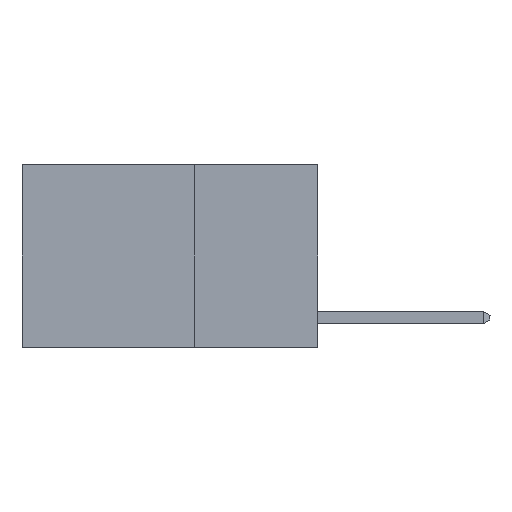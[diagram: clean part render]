
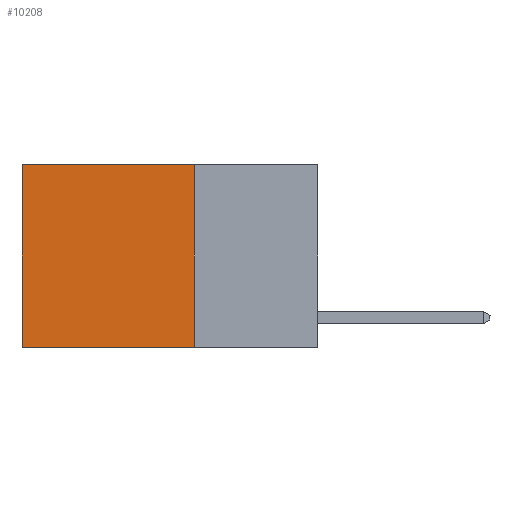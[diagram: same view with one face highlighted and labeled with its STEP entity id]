
A CAD part, left-side view. The second image highlights one B-rep face of the part: STEP entity #10208.
In plain terms, the highlighted planar face has unit normal (-1, 0, 0).
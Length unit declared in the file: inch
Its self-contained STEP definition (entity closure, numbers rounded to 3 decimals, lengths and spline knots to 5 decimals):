
#796 = LINE ( 'NONE', #3553, #7300 ) ;
#932 = VERTEX_POINT ( 'NONE', #9899 ) ;
#1137 = VECTOR ( 'NONE', #1715, 39.37008 ) ;
#1158 = LINE ( 'NONE', #10447, #4116 ) ;
#1715 = DIRECTION ( 'NONE',  ( 0., 0., -1. ) ) ;
#1800 = CARTESIAN_POINT ( 'NONE',  ( 0.2625, 0.25, 0. ) ) ;
#2267 = LINE ( 'NONE', #8555, #8526 ) ;
#2397 = DIRECTION ( 'NONE',  ( 1., 0., 0. ) ) ;
#3430 = EDGE_CURVE ( 'NONE', #6355, #932, #2267, .T. ) ;
#3553 = CARTESIAN_POINT ( 'NONE',  ( 0.2625, 0.6, 0. ) ) ;
#3679 = ORIENTED_EDGE ( 'NONE', *, *, #3430, .T. ) ;
#3944 = PLANE ( 'NONE',  #4107 ) ;
#4002 = FACE_OUTER_BOUND ( 'NONE', #10683, .T. ) ;
#4107 = AXIS2_PLACEMENT_3D ( 'NONE', #7612, #2397, #5086 ) ;
#4116 = VECTOR ( 'NONE', #8551, 39.37008 ) ;
#5086 = DIRECTION ( 'NONE',  ( 0., 0., -1. ) ) ;
#5306 = EDGE_CURVE ( 'NONE', #6355, #10913, #8979, .T. ) ;
#5366 = EDGE_CURVE ( 'NONE', #932, #8522, #796, .T. ) ;
#6355 = VERTEX_POINT ( 'NONE', #1800 ) ;
#6560 = CARTESIAN_POINT ( 'NONE',  ( 0.2625, 0.25, -0.37 ) ) ;
#6925 = ORIENTED_EDGE ( 'NONE', *, *, #5366, .T. ) ;
#7300 = VECTOR ( 'NONE', #10950, 39.37008 ) ;
#7612 = CARTESIAN_POINT ( 'NONE',  ( 0.2625, 0.25, 0. ) ) ;
#7735 = DIRECTION ( 'NONE',  ( 0., 1., 0. ) ) ;
#8126 = CARTESIAN_POINT ( 'NONE',  ( 0.2625, 0.6, -0.37 ) ) ;
#8301 = ORIENTED_EDGE ( 'NONE', *, *, #10554, .F. ) ;
#8522 = VERTEX_POINT ( 'NONE', #8126 ) ;
#8526 = VECTOR ( 'NONE', #7735, 39.37008 ) ;
#8551 = DIRECTION ( 'NONE',  ( 0., 1., 0. ) ) ;
#8555 = CARTESIAN_POINT ( 'NONE',  ( 0.2625, 0.25, 0. ) ) ;
#8979 = LINE ( 'NONE', #10892, #1137 ) ;
#9899 = CARTESIAN_POINT ( 'NONE',  ( 0.2625, 0.6, 0. ) ) ;
#10208 = ADVANCED_FACE ( 'NONE', ( #4002 ), #3944, .F. ) ;
#10447 = CARTESIAN_POINT ( 'NONE',  ( 0.2625, 0.25, -0.37 ) ) ;
#10554 = EDGE_CURVE ( 'NONE', #10913, #8522, #1158, .T. ) ;
#10683 = EDGE_LOOP ( 'NONE', ( #6925, #8301, #11391, #3679 ) ) ;
#10892 = CARTESIAN_POINT ( 'NONE',  ( 0.2625, 0.25, 0. ) ) ;
#10913 = VERTEX_POINT ( 'NONE', #6560 ) ;
#10950 = DIRECTION ( 'NONE',  ( 0., 0., -1. ) ) ;
#11391 = ORIENTED_EDGE ( 'NONE', *, *, #5306, .F. ) ;
